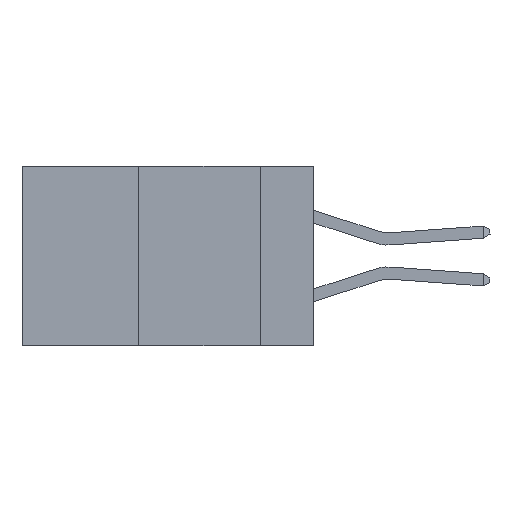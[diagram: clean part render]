
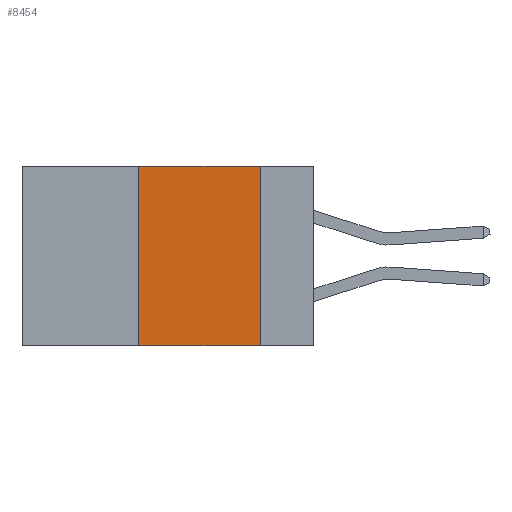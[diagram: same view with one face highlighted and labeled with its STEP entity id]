
A CAD part, left-side view. The second image highlights one B-rep face of the part: STEP entity #8454.
In plain terms, the highlighted planar face has unit normal (-1, 0, 0).
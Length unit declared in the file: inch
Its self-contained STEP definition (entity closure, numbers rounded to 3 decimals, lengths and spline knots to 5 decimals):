
#660 = DIRECTION ( 'NONE',  ( 1., 0., 0. ) ) ;
#766 = LINE ( 'NONE', #18874, #6704 ) ;
#949 = EDGE_CURVE ( 'NONE', #6168, #2483, #766, .T. ) ;
#2483 = VERTEX_POINT ( 'NONE', #12011 ) ;
#4317 = LINE ( 'NONE', #4549, #17557 ) ;
#4549 = CARTESIAN_POINT ( 'NONE',  ( 0., 0.6, -0.37 ) ) ;
#6168 = VERTEX_POINT ( 'NONE', #9853 ) ;
#6674 = AXIS2_PLACEMENT_3D ( 'NONE', #22159, #660, #7809 ) ;
#6704 = VECTOR ( 'NONE', #7914, 39.37008 ) ;
#7139 = LINE ( 'NONE', #10546, #16768 ) ;
#7809 = DIRECTION ( 'NONE',  ( 0., 0., -1. ) ) ;
#7880 = ORIENTED_EDGE ( 'NONE', *, *, #7918, .T. ) ;
#7914 = DIRECTION ( 'NONE',  ( 0., -1., 0. ) ) ;
#7918 = EDGE_CURVE ( 'NONE', #11772, #10581, #4317, .T. ) ;
#8454 = ADVANCED_FACE ( 'NONE', ( #20409 ), #16998, .F. ) ;
#8767 = EDGE_LOOP ( 'NONE', ( #23163, #12565, #21135, #7880 ) ) ;
#9853 = CARTESIAN_POINT ( 'NONE',  ( 0., 0.36, 0. ) ) ;
#10173 = DIRECTION ( 'NONE',  ( 0., -1., 0. ) ) ;
#10546 = CARTESIAN_POINT ( 'NONE',  ( 0., 0.11, 0. ) ) ;
#10581 = VERTEX_POINT ( 'NONE', #14915 ) ;
#11307 = LINE ( 'NONE', #16709, #14183 ) ;
#11772 = VERTEX_POINT ( 'NONE', #17866 ) ;
#12011 = CARTESIAN_POINT ( 'NONE',  ( 0., 0.11, 0. ) ) ;
#12565 = ORIENTED_EDGE ( 'NONE', *, *, #949, .F. ) ;
#14183 = VECTOR ( 'NONE', #16481, 39.37008 ) ;
#14915 = CARTESIAN_POINT ( 'NONE',  ( 0., 0.11, -0.37 ) ) ;
#15951 = DIRECTION ( 'NONE',  ( 0., 0., -1. ) ) ;
#16481 = DIRECTION ( 'NONE',  ( 0., 0., 1. ) ) ;
#16709 = CARTESIAN_POINT ( 'NONE',  ( 0., 0.36, 0. ) ) ;
#16768 = VECTOR ( 'NONE', #15951, 39.37008 ) ;
#16998 = PLANE ( 'NONE',  #6674 ) ;
#17557 = VECTOR ( 'NONE', #10173, 39.37008 ) ;
#17866 = CARTESIAN_POINT ( 'NONE',  ( 0., 0.36, -0.37 ) ) ;
#18721 = EDGE_CURVE ( 'NONE', #11772, #6168, #11307, .T. ) ;
#18874 = CARTESIAN_POINT ( 'NONE',  ( 0., 0.6, 0. ) ) ;
#19133 = EDGE_CURVE ( 'NONE', #2483, #10581, #7139, .T. ) ;
#20409 = FACE_OUTER_BOUND ( 'NONE', #8767, .T. ) ;
#21135 = ORIENTED_EDGE ( 'NONE', *, *, #18721, .F. ) ;
#22159 = CARTESIAN_POINT ( 'NONE',  ( 0., 0.6, 0. ) ) ;
#23163 = ORIENTED_EDGE ( 'NONE', *, *, #19133, .F. ) ;
